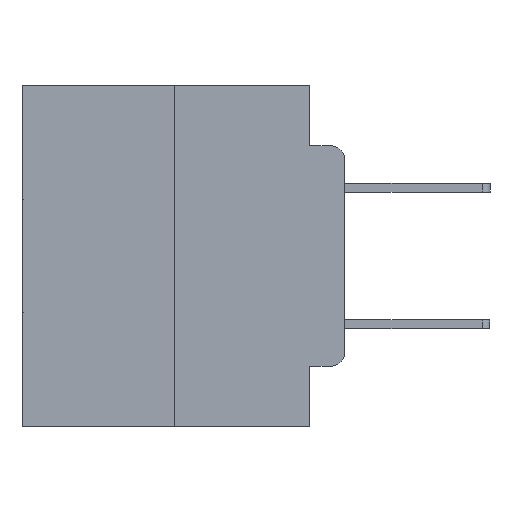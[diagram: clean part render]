
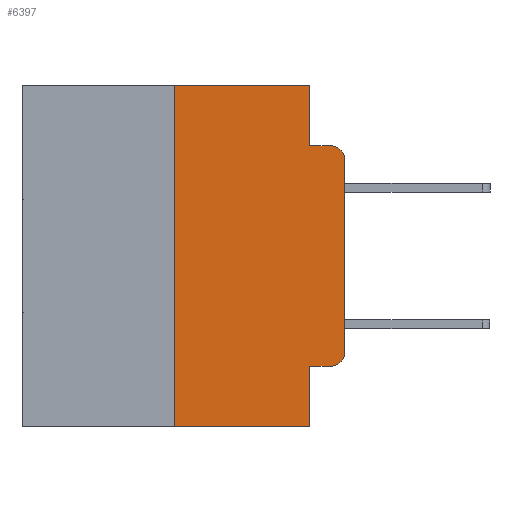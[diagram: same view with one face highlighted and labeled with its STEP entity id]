
A CAD part, left-side view. The second image highlights one B-rep face of the part: STEP entity #6397.
In plain terms, the highlighted planar face has unit normal (-1, 0, 0).
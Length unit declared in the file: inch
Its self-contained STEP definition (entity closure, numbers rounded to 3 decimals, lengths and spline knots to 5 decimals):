
#392 = EDGE_CURVE ( 'NONE', #13055, #11727, #2061, .T. ) ;
#630 = AXIS2_PLACEMENT_3D ( 'NONE', #22216, #8736, #26302 ) ;
#707 = VERTEX_POINT ( 'NONE', #8203 ) ;
#918 = EDGE_CURVE ( 'NONE', #16091, #14789, #26333, .T. ) ;
#1387 = DIRECTION ( 'NONE',  ( -1., 0., 0. ) ) ;
#1599 = VERTEX_POINT ( 'NONE', #16586 ) ;
#1861 = CARTESIAN_POINT ( 'NONE',  ( 0., 0.473, 0. ) ) ;
#2061 = LINE ( 'NONE', #4048, #23522 ) ;
#2153 = EDGE_CURVE ( 'NONE', #8977, #15191, #19952, .T. ) ;
#2216 = DIRECTION ( 'NONE',  ( 0., -1., 0. ) ) ;
#2528 = DIRECTION ( 'NONE',  ( 0., -1., 0. ) ) ;
#2724 = CARTESIAN_POINT ( 'NONE',  ( 0., 0.051, -0.4115 ) ) ;
#2801 = VECTOR ( 'NONE', #26229, 39.37008 ) ;
#3197 = DIRECTION ( 'NONE',  ( 0., -1., 0. ) ) ;
#3545 = CARTESIAN_POINT ( 'NONE',  ( 0., 0.051, -0.5 ) ) ;
#3916 = CARTESIAN_POINT ( 'NONE',  ( 0., 0.02, -0.4115 ) ) ;
#4048 = CARTESIAN_POINT ( 'NONE',  ( 0., 0.051, -0.4115 ) ) ;
#4061 = DIRECTION ( 'NONE',  ( 1., 0., 0. ) ) ;
#4068 = LINE ( 'NONE', #25961, #20014 ) ;
#4074 = CARTESIAN_POINT ( 'NONE',  ( 0., 0.051, 0. ) ) ;
#4942 = CARTESIAN_POINT ( 'NONE',  ( 0., 0.473, 0. ) ) ;
#5273 = EDGE_CURVE ( 'NONE', #8441, #20273, #14061, .T. ) ;
#5305 = AXIS2_PLACEMENT_3D ( 'NONE', #14144, #1387, #16223 ) ;
#5312 = EDGE_CURVE ( 'NONE', #8441, #8977, #7145, .T. ) ;
#6397 = ADVANCED_FACE ( 'NONE', ( #26218 ), #14583, .F. ) ;
#6728 = CARTESIAN_POINT ( 'NONE',  ( 0., 0.473, -0.5 ) ) ;
#7145 = LINE ( 'NONE', #26145, #2801 ) ;
#7619 = EDGE_CURVE ( 'NONE', #11727, #707, #24559, .T. ) ;
#8203 = CARTESIAN_POINT ( 'NONE',  ( 0., 0., -0.3915 ) ) ;
#8441 = VERTEX_POINT ( 'NONE', #10568 ) ;
#8736 = DIRECTION ( 'NONE',  ( -1., 0., 0. ) ) ;
#8977 = VERTEX_POINT ( 'NONE', #26752 ) ;
#9206 = DIRECTION ( 'NONE',  ( 0., -1., 0. ) ) ;
#9582 = EDGE_CURVE ( 'NONE', #15191, #1599, #4068, .T. ) ;
#10124 = LINE ( 'NONE', #15571, #25770 ) ;
#10568 = CARTESIAN_POINT ( 'NONE',  ( 0., 0.25, -0.5 ) ) ;
#11638 = ORIENTED_EDGE ( 'NONE', *, *, #15699, .T. ) ;
#11716 = ORIENTED_EDGE ( 'NONE', *, *, #918, .T. ) ;
#11727 = VERTEX_POINT ( 'NONE', #3916 ) ;
#11978 = ORIENTED_EDGE ( 'NONE', *, *, #25170, .F. ) ;
#12141 = ORIENTED_EDGE ( 'NONE', *, *, #9582, .F. ) ;
#12207 = CARTESIAN_POINT ( 'NONE',  ( 0., 0., 0. ) ) ;
#12209 = ORIENTED_EDGE ( 'NONE', *, *, #2153, .F. ) ;
#12385 = ORIENTED_EDGE ( 'NONE', *, *, #5312, .F. ) ;
#12472 = ORIENTED_EDGE ( 'NONE', *, *, #23291, .F. ) ;
#12678 = ORIENTED_EDGE ( 'NONE', *, *, #392, .T. ) ;
#12837 = ORIENTED_EDGE ( 'NONE', *, *, #7619, .T. ) ;
#13055 = VERTEX_POINT ( 'NONE', #2724 ) ;
#13463 = ORIENTED_EDGE ( 'NONE', *, *, #5273, .T. ) ;
#13486 = DIRECTION ( 'NONE',  ( 0., 0., -1. ) ) ;
#13818 = DIRECTION ( 'NONE',  ( 0., 0., -1. ) ) ;
#14061 = LINE ( 'NONE', #6728, #18836 ) ;
#14144 = CARTESIAN_POINT ( 'NONE',  ( 0., 0.02, -0.3915 ) ) ;
#14447 = AXIS2_PLACEMENT_3D ( 'NONE', #1861, #4061, #18650 ) ;
#14568 = VECTOR ( 'NONE', #2216, 39.37008 ) ;
#14583 = PLANE ( 'NONE',  #14447 ) ;
#14789 = VERTEX_POINT ( 'NONE', #21186 ) ;
#15191 = VERTEX_POINT ( 'NONE', #4074 ) ;
#15571 = CARTESIAN_POINT ( 'NONE',  ( 0., 0.051, 0. ) ) ;
#15699 = EDGE_CURVE ( 'NONE', #707, #16091, #26559, .T. ) ;
#16091 = VERTEX_POINT ( 'NONE', #19525 ) ;
#16223 = DIRECTION ( 'NONE',  ( 0., 0., -1. ) ) ;
#16586 = CARTESIAN_POINT ( 'NONE',  ( 0., 0.051, -0.0885 ) ) ;
#18650 = DIRECTION ( 'NONE',  ( 0., 0., -1. ) ) ;
#18836 = VECTOR ( 'NONE', #2528, 39.37008 ) ;
#19525 = CARTESIAN_POINT ( 'NONE',  ( 0., 0., -0.1085 ) ) ;
#19575 = VECTOR ( 'NONE', #3197, 39.37008 ) ;
#19801 = CARTESIAN_POINT ( 'NONE',  ( 0., 0.051, -0.0885 ) ) ;
#19952 = LINE ( 'NONE', #4942, #14568 ) ;
#20014 = VECTOR ( 'NONE', #13818, 39.37008 ) ;
#20188 = LINE ( 'NONE', #19801, #19575 ) ;
#20273 = VERTEX_POINT ( 'NONE', #3545 ) ;
#20543 = VECTOR ( 'NONE', #26410, 39.37008 ) ;
#20760 = EDGE_LOOP ( 'NONE', ( #11638, #11716, #11978, #12141, #12209, #12385, #13463, #12472, #12678, #12837 ) ) ;
#21186 = CARTESIAN_POINT ( 'NONE',  ( 0., 0.02, -0.0885 ) ) ;
#22216 = CARTESIAN_POINT ( 'NONE',  ( 0., 0.02, -0.1085 ) ) ;
#23291 = EDGE_CURVE ( 'NONE', #13055, #20273, #10124, .T. ) ;
#23522 = VECTOR ( 'NONE', #9206, 39.37008 ) ;
#24559 = CIRCLE ( 'NONE', #5305, 0.02 ) ;
#25170 = EDGE_CURVE ( 'NONE', #1599, #14789, #20188, .T. ) ;
#25770 = VECTOR ( 'NONE', #13486, 39.37008 ) ;
#25961 = CARTESIAN_POINT ( 'NONE',  ( 0., 0.051, 0. ) ) ;
#26145 = CARTESIAN_POINT ( 'NONE',  ( 0., 0.25, 0. ) ) ;
#26218 = FACE_OUTER_BOUND ( 'NONE', #20760, .T. ) ;
#26229 = DIRECTION ( 'NONE',  ( 0., 0., 1. ) ) ;
#26302 = DIRECTION ( 'NONE',  ( 0., 0., -1. ) ) ;
#26333 = CIRCLE ( 'NONE', #630, 0.02 ) ;
#26410 = DIRECTION ( 'NONE',  ( 0., 0., 1. ) ) ;
#26559 = LINE ( 'NONE', #12207, #20543 ) ;
#26752 = CARTESIAN_POINT ( 'NONE',  ( 0., 0.25, 0. ) ) ;
